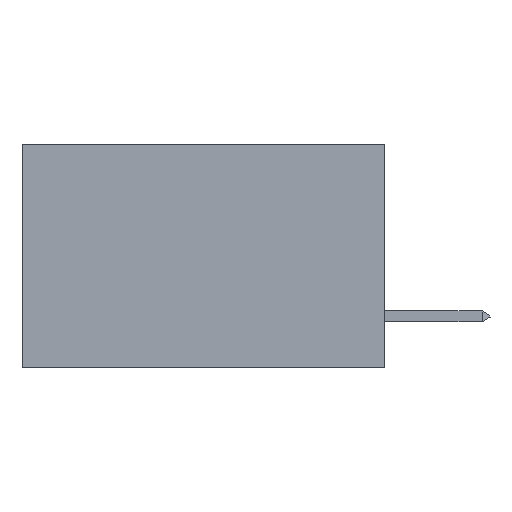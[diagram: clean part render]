
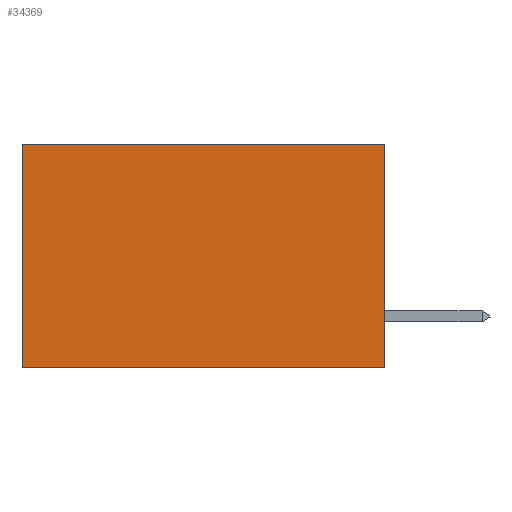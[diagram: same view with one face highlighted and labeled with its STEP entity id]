
A CAD part, left-side view. The second image highlights one B-rep face of the part: STEP entity #34369.
In plain terms, the highlighted planar face has unit normal (-1, 0, 0).
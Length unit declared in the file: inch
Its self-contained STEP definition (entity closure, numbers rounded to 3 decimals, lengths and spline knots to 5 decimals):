
#71 = AXIS2_PLACEMENT_3D ( 'NONE', #23026, #3055, #33076 ) ;
#171 = ORIENTED_EDGE ( 'NONE', *, *, #31354, .F. ) ;
#955 = CARTESIAN_POINT ( 'NONE',  ( 0.2875, 0.6, -0.37 ) ) ;
#1541 = ORIENTED_EDGE ( 'NONE', *, *, #33042, .T. ) ;
#1739 = DIRECTION ( 'NONE',  ( 0., 0., -1. ) ) ;
#2534 = VERTEX_POINT ( 'NONE', #955 ) ;
#3055 = DIRECTION ( 'NONE',  ( 1., 0., 0. ) ) ;
#3941 = VECTOR ( 'NONE', #10637, 39.37008 ) ;
#3960 = CARTESIAN_POINT ( 'NONE',  ( 0.2875, 0., 0. ) ) ;
#5702 = EDGE_CURVE ( 'NONE', #42186, #2534, #36501, .T. ) ;
#6482 = LINE ( 'NONE', #3960, #3941 ) ;
#6635 = LINE ( 'NONE', #28072, #38453 ) ;
#10020 = FACE_OUTER_BOUND ( 'NONE', #40893, .T. ) ;
#10637 = DIRECTION ( 'NONE',  ( 0., 1., 0. ) ) ;
#11152 = VERTEX_POINT ( 'NONE', #32599 ) ;
#13647 = EDGE_CURVE ( 'NONE', #11152, #35976, #6635, .T. ) ;
#15285 = ORIENTED_EDGE ( 'NONE', *, *, #13647, .F. ) ;
#16282 = PLANE ( 'NONE',  #71 ) ;
#21659 = CARTESIAN_POINT ( 'NONE',  ( 0.2875, 0.6, 0. ) ) ;
#23026 = CARTESIAN_POINT ( 'NONE',  ( 0.2875, 0., 0. ) ) ;
#23620 = CARTESIAN_POINT ( 'NONE',  ( 0.2875, 0., -0.37 ) ) ;
#27052 = VECTOR ( 'NONE', #30334, 39.37008 ) ;
#28072 = CARTESIAN_POINT ( 'NONE',  ( 0.2875, 0., 0. ) ) ;
#28610 = LINE ( 'NONE', #23620, #27052 ) ;
#30334 = DIRECTION ( 'NONE',  ( 0., 1., 0. ) ) ;
#31354 = EDGE_CURVE ( 'NONE', #35976, #2534, #28610, .T. ) ;
#32599 = CARTESIAN_POINT ( 'NONE',  ( 0.2875, 0., 0. ) ) ;
#33042 = EDGE_CURVE ( 'NONE', #11152, #42186, #6482, .T. ) ;
#33076 = DIRECTION ( 'NONE',  ( 0., 0., -1. ) ) ;
#34369 = ADVANCED_FACE ( 'NONE', ( #10020 ), #16282, .F. ) ;
#34587 = ORIENTED_EDGE ( 'NONE', *, *, #5702, .T. ) ;
#35976 = VERTEX_POINT ( 'NONE', #40605 ) ;
#36501 = LINE ( 'NONE', #41239, #38014 ) ;
#38014 = VECTOR ( 'NONE', #1739, 39.37008 ) ;
#38453 = VECTOR ( 'NONE', #41825, 39.37008 ) ;
#40605 = CARTESIAN_POINT ( 'NONE',  ( 0.2875, 0., -0.37 ) ) ;
#40893 = EDGE_LOOP ( 'NONE', ( #34587, #171, #15285, #1541 ) ) ;
#41239 = CARTESIAN_POINT ( 'NONE',  ( 0.2875, 0.6, 0. ) ) ;
#41825 = DIRECTION ( 'NONE',  ( 0., 0., -1. ) ) ;
#42186 = VERTEX_POINT ( 'NONE', #21659 ) ;
